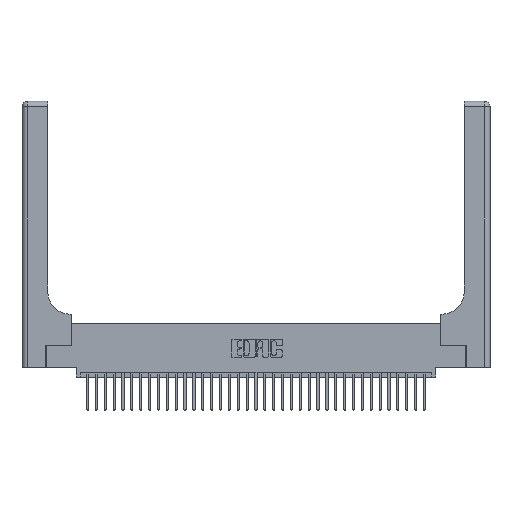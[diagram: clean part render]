
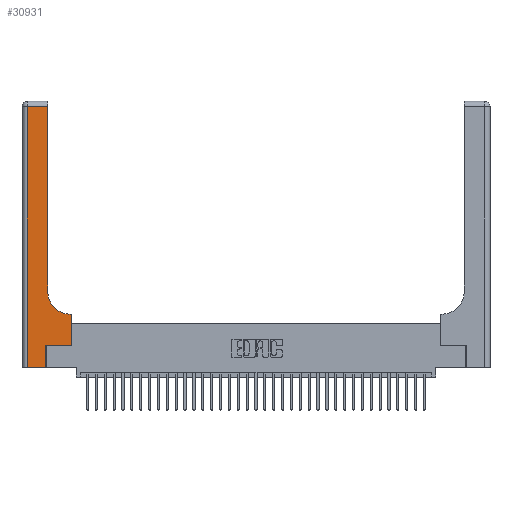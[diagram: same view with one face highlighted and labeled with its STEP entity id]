
A CAD part, top view. The second image highlights one B-rep face of the part: STEP entity #30931.
In plain terms, the highlighted planar face has unit normal (0, 0, 1).
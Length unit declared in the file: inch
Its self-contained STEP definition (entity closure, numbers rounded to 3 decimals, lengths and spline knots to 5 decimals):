
#659 = EDGE_CURVE ( 'NONE', #34064, #7562, #31583, .T. ) ;
#925 = CARTESIAN_POINT ( 'NONE',  ( 0.5415, 0.6, 0.37 ) ) ;
#1123 = CARTESIAN_POINT ( 'NONE',  ( 0., 3., 0.37 ) ) ;
#1196 = ORIENTED_EDGE ( 'NONE', *, *, #35206, .T. ) ;
#1421 = FACE_OUTER_BOUND ( 'NONE', #7738, .T. ) ;
#1492 = CARTESIAN_POINT ( 'NONE',  ( 0.269, 0.25, 0.37 ) ) ;
#1498 = CARTESIAN_POINT ( 'NONE',  ( 0.269, 0.25, 0.37 ) ) ;
#1787 = ORIENTED_EDGE ( 'NONE', *, *, #26605, .T. ) ;
#2113 = AXIS2_PLACEMENT_3D ( 'NONE', #1123, #3920, #23631 ) ;
#2737 = EDGE_CURVE ( 'NONE', #12068, #11883, #19188, .T. ) ;
#3160 = ORIENTED_EDGE ( 'NONE', *, *, #23105, .T. ) ;
#3920 = DIRECTION ( 'NONE',  ( 0., 0., -1. ) ) ;
#4148 = EDGE_CURVE ( 'NONE', #28307, #27581, #21776, .T. ) ;
#4238 = VECTOR ( 'NONE', #35544, 39.37008 ) ;
#4242 = LINE ( 'NONE', #12579, #33238 ) ;
#4303 = DIRECTION ( 'NONE',  ( 1., 0., 0. ) ) ;
#4714 = DIRECTION ( 'NONE',  ( -1., 0., 0. ) ) ;
#4837 = VECTOR ( 'NONE', #18924, 39.37008 ) ;
#5805 = VERTEX_POINT ( 'NONE', #30391 ) ;
#6219 = VECTOR ( 'NONE', #12525, 39.37008 ) ;
#6225 = CARTESIAN_POINT ( 'NONE',  ( 0.5415, 0.85, 0.37 ) ) ;
#6312 = ORIENTED_EDGE ( 'NONE', *, *, #10000, .T. ) ;
#7562 = VERTEX_POINT ( 'NONE', #22225 ) ;
#7738 = EDGE_LOOP ( 'NONE', ( #3160, #6312, #11908, #1787, #22981, #1196, #12276, #14304, #22935 ) ) ;
#9033 = DIRECTION ( 'NONE',  ( 1., 0., 0. ) ) ;
#9430 = EDGE_CURVE ( 'NONE', #27581, #18827, #11707, .T. ) ;
#10000 = EDGE_CURVE ( 'NONE', #5805, #34064, #35238, .T. ) ;
#11036 = CIRCLE ( 'NONE', #23944, 0.25 ) ;
#11707 = LINE ( 'NONE', #32719, #31506 ) ;
#11883 = VERTEX_POINT ( 'NONE', #1492 ) ;
#11908 = ORIENTED_EDGE ( 'NONE', *, *, #659, .T. ) ;
#12068 = VERTEX_POINT ( 'NONE', #24716 ) ;
#12276 = ORIENTED_EDGE ( 'NONE', *, *, #4148, .T. ) ;
#12525 = DIRECTION ( 'NONE',  ( -1., 0., 0. ) ) ;
#12579 = CARTESIAN_POINT ( 'NONE',  ( 0.2915, 3., 0.37 ) ) ;
#13223 = CARTESIAN_POINT ( 'NONE',  ( 0., 0., 0.37 ) ) ;
#13826 = DIRECTION ( 'NONE',  ( 0., 1., 0. ) ) ;
#14221 = VECTOR ( 'NONE', #13826, 39.37008 ) ;
#14304 = ORIENTED_EDGE ( 'NONE', *, *, #9430, .T. ) ;
#17474 = VECTOR ( 'NONE', #27927, 39.37008 ) ;
#18827 = VERTEX_POINT ( 'NONE', #925 ) ;
#18924 = DIRECTION ( 'NONE',  ( 1., 0., 0. ) ) ;
#19188 = LINE ( 'NONE', #32248, #4238 ) ;
#20779 = PLANE ( 'NONE',  #2113 ) ;
#21776 = LINE ( 'NONE', #30576, #14221 ) ;
#22170 = VECTOR ( 'NONE', #4303, 39.37008 ) ;
#22225 = CARTESIAN_POINT ( 'NONE',  ( 0.06, 0., 0.37 ) ) ;
#22935 = ORIENTED_EDGE ( 'NONE', *, *, #25918, .T. ) ;
#22981 = ORIENTED_EDGE ( 'NONE', *, *, #2737, .T. ) ;
#23105 = EDGE_CURVE ( 'NONE', #28472, #5805, #4242, .T. ) ;
#23541 = CARTESIAN_POINT ( 'NONE',  ( 0.5585, 0.25, 0.37 ) ) ;
#23631 = DIRECTION ( 'NONE',  ( -1., 0., 0. ) ) ;
#23944 = AXIS2_PLACEMENT_3D ( 'NONE', #6225, #25934, #9033 ) ;
#24716 = CARTESIAN_POINT ( 'NONE',  ( 0.269, 0., 0.37 ) ) ;
#25918 = EDGE_CURVE ( 'NONE', #18827, #28472, #11036, .T. ) ;
#25934 = DIRECTION ( 'NONE',  ( 0., 0., -1. ) ) ;
#26605 = EDGE_CURVE ( 'NONE', #7562, #12068, #28171, .T. ) ;
#26722 = CARTESIAN_POINT ( 'NONE',  ( 0., 2.94, 0.37 ) ) ;
#27581 = VERTEX_POINT ( 'NONE', #28935 ) ;
#27927 = DIRECTION ( 'NONE',  ( 0., -1., 0. ) ) ;
#28171 = LINE ( 'NONE', #13223, #4837 ) ;
#28307 = VERTEX_POINT ( 'NONE', #23541 ) ;
#28472 = VERTEX_POINT ( 'NONE', #32674 ) ;
#28935 = CARTESIAN_POINT ( 'NONE',  ( 0.5585, 0.6, 0.37 ) ) ;
#30391 = CARTESIAN_POINT ( 'NONE',  ( 0.2915, 2.94, 0.37 ) ) ;
#30462 = LINE ( 'NONE', #1498, #22170 ) ;
#30576 = CARTESIAN_POINT ( 'NONE',  ( 0.5585, 0.25, 0.37 ) ) ;
#30931 = ADVANCED_FACE ( 'NONE', ( #1421 ), #20779, .F. ) ;
#31506 = VECTOR ( 'NONE', #4714, 39.37008 ) ;
#31583 = LINE ( 'NONE', #35294, #17474 ) ;
#32248 = CARTESIAN_POINT ( 'NONE',  ( 0.269, 0., 0.37 ) ) ;
#32263 = DIRECTION ( 'NONE',  ( 0., 1., 0. ) ) ;
#32674 = CARTESIAN_POINT ( 'NONE',  ( 0.2915, 0.85, 0.37 ) ) ;
#32719 = CARTESIAN_POINT ( 'NONE',  ( 0.2915, 0.6, 0.37 ) ) ;
#33238 = VECTOR ( 'NONE', #32263, 39.37008 ) ;
#33664 = CARTESIAN_POINT ( 'NONE',  ( 0.06, 2.94, 0.37 ) ) ;
#34064 = VERTEX_POINT ( 'NONE', #33664 ) ;
#35206 = EDGE_CURVE ( 'NONE', #11883, #28307, #30462, .T. ) ;
#35238 = LINE ( 'NONE', #26722, #6219 ) ;
#35294 = CARTESIAN_POINT ( 'NONE',  ( 0.06, 3., 0.37 ) ) ;
#35544 = DIRECTION ( 'NONE',  ( 0., 1., 0. ) ) ;
